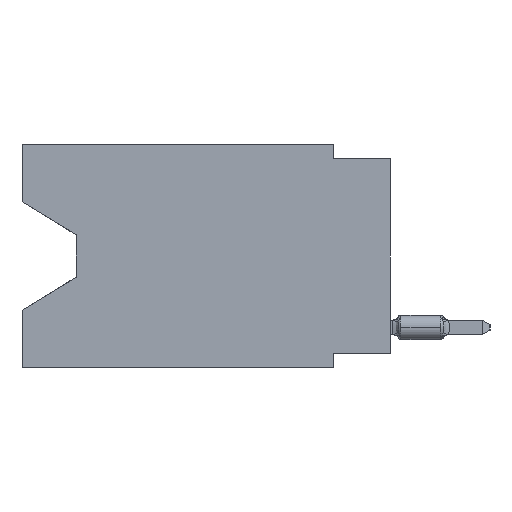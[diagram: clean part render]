
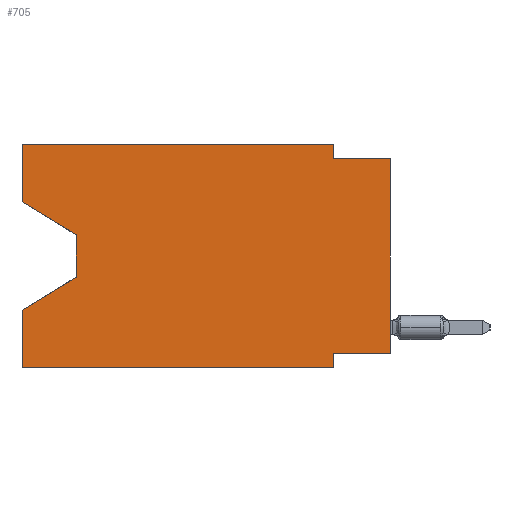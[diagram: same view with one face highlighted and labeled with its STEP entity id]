
A CAD part, left-side view. The second image highlights one B-rep face of the part: STEP entity #705.
In plain terms, the highlighted planar face has unit normal (-1, 0, 0).
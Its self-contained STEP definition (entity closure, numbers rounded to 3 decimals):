
#705 = ADVANCED_FACE ( 'NONE', ( #65402 ), #27358, .F. ) ;
#1265 = VERTEX_POINT ( 'NONE', #49003 ) ;
#1411 = DIRECTION ( 'NONE',  ( 0., 0.855, -0.519 ) ) ;
#3515 = ORIENTED_EDGE ( 'NONE', *, *, #37311, .F. ) ;
#3719 = VECTOR ( 'NONE', #31728, 1000. ) ;
#6799 = LINE ( 'NONE', #12261, #25648 ) ;
#6961 = DIRECTION ( 'NONE',  ( 0., 0., -1. ) ) ;
#7581 = VECTOR ( 'NONE', #49645, 1000. ) ;
#8036 = CARTESIAN_POINT ( 'NONE',  ( 0., 13.97, -4.013 ) ) ;
#8520 = CARTESIAN_POINT ( 'NONE',  ( 0., 0., -0.635 ) ) ;
#9161 = EDGE_CURVE ( 'NONE', #67876, #71283, #30397, .T. ) ;
#9735 = VECTOR ( 'NONE', #6961, 1000. ) ;
#10571 = VERTEX_POINT ( 'NONE', #27828 ) ;
#12261 = CARTESIAN_POINT ( 'NONE',  ( 0., 0., 0. ) ) ;
#13777 = LINE ( 'NONE', #39288, #30095 ) ;
#14606 = VECTOR ( 'NONE', #23085, 1000. ) ;
#18423 = CARTESIAN_POINT ( 'NONE',  ( 0., 2.54, -9.906 ) ) ;
#18694 = LINE ( 'NONE', #44208, #9735 ) ;
#18821 = DIRECTION ( 'NONE',  ( 0., 0., -1. ) ) ;
#19104 = EDGE_CURVE ( 'NONE', #69450, #24934, #51609, .T. ) ;
#19611 = VECTOR ( 'NONE', #56331, 1000. ) ;
#19789 = VERTEX_POINT ( 'NONE', #56767 ) ;
#19826 = LINE ( 'NONE', #52847, #44506 ) ;
#21110 = DIRECTION ( 'NONE',  ( 1., 0., 0. ) ) ;
#23085 = DIRECTION ( 'NONE',  ( 0., 0., 1. ) ) ;
#23107 = ORIENTED_EDGE ( 'NONE', *, *, #48352, .T. ) ;
#24934 = VERTEX_POINT ( 'NONE', #54154 ) ;
#25648 = VECTOR ( 'NONE', #56995, 1000. ) ;
#26311 = EDGE_CURVE ( 'NONE', #45090, #24934, #80147, .T. ) ;
#27358 = PLANE ( 'NONE',  #37511 ) ;
#27828 = CARTESIAN_POINT ( 'NONE',  ( 0., 2.54, -9.271 ) ) ;
#28147 = LINE ( 'NONE', #8520, #42936 ) ;
#29198 = ORIENTED_EDGE ( 'NONE', *, *, #49040, .F. ) ;
#30003 = CARTESIAN_POINT ( 'NONE',  ( 0., 13.97, -4.013 ) ) ;
#30095 = VECTOR ( 'NONE', #63555, 1000. ) ;
#30397 = LINE ( 'NONE', #69262, #7581 ) ;
#30816 = ORIENTED_EDGE ( 'NONE', *, *, #56239, .F. ) ;
#31728 = DIRECTION ( 'NONE',  ( 0., 1., 0. ) ) ;
#34284 = ORIENTED_EDGE ( 'NONE', *, *, #78993, .F. ) ;
#34293 = ORIENTED_EDGE ( 'NONE', *, *, #9161, .T. ) ;
#37311 = EDGE_CURVE ( 'NONE', #48006, #76454, #18694, .T. ) ;
#37511 = AXIS2_PLACEMENT_3D ( 'NONE', #78361, #21110, #46625 ) ;
#38422 = LINE ( 'NONE', #63903, #3719 ) ;
#39288 = CARTESIAN_POINT ( 'NONE',  ( 0., 16.383, -9.906 ) ) ;
#41454 = CARTESIAN_POINT ( 'NONE',  ( 0., 16.383, -2.546 ) ) ;
#41737 = DIRECTION ( 'NONE',  ( 0., 0., -1. ) ) ;
#42146 = LINE ( 'NONE', #30003, #52221 ) ;
#42936 = VECTOR ( 'NONE', #72458, 1000. ) ;
#43181 = EDGE_CURVE ( 'NONE', #1265, #10571, #38422, .T. ) ;
#44208 = CARTESIAN_POINT ( 'NONE',  ( 0., 2.54, 0. ) ) ;
#44506 = VECTOR ( 'NONE', #52015, 1000. ) ;
#45090 = VERTEX_POINT ( 'NONE', #72975 ) ;
#46625 = DIRECTION ( 'NONE',  ( 0., 0., -1. ) ) ;
#47156 = ORIENTED_EDGE ( 'NONE', *, *, #19104, .T. ) ;
#48006 = VERTEX_POINT ( 'NONE', #62706 ) ;
#48352 = EDGE_CURVE ( 'NONE', #71283, #69450, #42146, .T. ) ;
#48355 = ORIENTED_EDGE ( 'NONE', *, *, #63281, .F. ) ;
#48427 = CARTESIAN_POINT ( 'NONE',  ( 0., 0., -0.635 ) ) ;
#49003 = CARTESIAN_POINT ( 'NONE',  ( 0., 0., -9.271 ) ) ;
#49040 = EDGE_CURVE ( 'NONE', #76454, #62012, #28147, .T. ) ;
#49645 = DIRECTION ( 'NONE',  ( 0., -0.855, -0.519 ) ) ;
#50204 = LINE ( 'NONE', #18423, #52951 ) ;
#50210 = CARTESIAN_POINT ( 'NONE',  ( 0., 16.383, 0. ) ) ;
#51609 = LINE ( 'NONE', #71209, #55314 ) ;
#52015 = DIRECTION ( 'NONE',  ( 0., -1., 0. ) ) ;
#52221 = VECTOR ( 'NONE', #41737, 1000. ) ;
#52847 = CARTESIAN_POINT ( 'NONE',  ( 0., 16.383, 0. ) ) ;
#52951 = VECTOR ( 'NONE', #18821, 1000. ) ;
#53704 = ORIENTED_EDGE ( 'NONE', *, *, #43181, .F. ) ;
#54053 = CARTESIAN_POINT ( 'NONE',  ( 0., 16.383, 0. ) ) ;
#54154 = CARTESIAN_POINT ( 'NONE',  ( 0., 16.383, -7.36 ) ) ;
#55314 = VECTOR ( 'NONE', #1411, 1000. ) ;
#56239 = EDGE_CURVE ( 'NONE', #67876, #73653, #80346, .T. ) ;
#56331 = DIRECTION ( 'NONE',  ( 0., 0., 1. ) ) ;
#56767 = CARTESIAN_POINT ( 'NONE',  ( 0., 2.54, -9.906 ) ) ;
#56995 = DIRECTION ( 'NONE',  ( 0., 0., 1. ) ) ;
#58154 = ORIENTED_EDGE ( 'NONE', *, *, #26311, .F. ) ;
#62012 = VERTEX_POINT ( 'NONE', #48427 ) ;
#62593 = CARTESIAN_POINT ( 'NONE',  ( 0., 16.383, 0. ) ) ;
#62706 = CARTESIAN_POINT ( 'NONE',  ( 0., 2.54, 0. ) ) ;
#62731 = ORIENTED_EDGE ( 'NONE', *, *, #71143, .T. ) ;
#63281 = EDGE_CURVE ( 'NONE', #10571, #19789, #50204, .T. ) ;
#63555 = DIRECTION ( 'NONE',  ( 0., -1., 0. ) ) ;
#63903 = CARTESIAN_POINT ( 'NONE',  ( 0., 0., -9.271 ) ) ;
#65402 = FACE_OUTER_BOUND ( 'NONE', #77469, .T. ) ;
#67876 = VERTEX_POINT ( 'NONE', #41454 ) ;
#69262 = CARTESIAN_POINT ( 'NONE',  ( 0., 16.383, -2.546 ) ) ;
#69450 = VERTEX_POINT ( 'NONE', #80085 ) ;
#71143 = EDGE_CURVE ( 'NONE', #1265, #62012, #6799, .T. ) ;
#71209 = CARTESIAN_POINT ( 'NONE',  ( 0., 13.97, -5.893 ) ) ;
#71283 = VERTEX_POINT ( 'NONE', #8036 ) ;
#72458 = DIRECTION ( 'NONE',  ( 0., -1., 0. ) ) ;
#72975 = CARTESIAN_POINT ( 'NONE',  ( 0., 16.383, -9.906 ) ) ;
#73653 = VERTEX_POINT ( 'NONE', #50210 ) ;
#75051 = EDGE_CURVE ( 'NONE', #45090, #19789, #13777, .T. ) ;
#76454 = VERTEX_POINT ( 'NONE', #81868 ) ;
#77469 = EDGE_LOOP ( 'NONE', ( #34293, #23107, #47156, #58154, #80347, #48355, #53704, #62731, #29198, #3515, #34284, #30816 ) ) ;
#78361 = CARTESIAN_POINT ( 'NONE',  ( 0., 16.383, 0. ) ) ;
#78993 = EDGE_CURVE ( 'NONE', #73653, #48006, #19826, .T. ) ;
#80085 = CARTESIAN_POINT ( 'NONE',  ( 0., 13.97, -5.893 ) ) ;
#80147 = LINE ( 'NONE', #62593, #19611 ) ;
#80346 = LINE ( 'NONE', #54053, #14606 ) ;
#80347 = ORIENTED_EDGE ( 'NONE', *, *, #75051, .T. ) ;
#81868 = CARTESIAN_POINT ( 'NONE',  ( 0., 2.54, -0.635 ) ) ;
